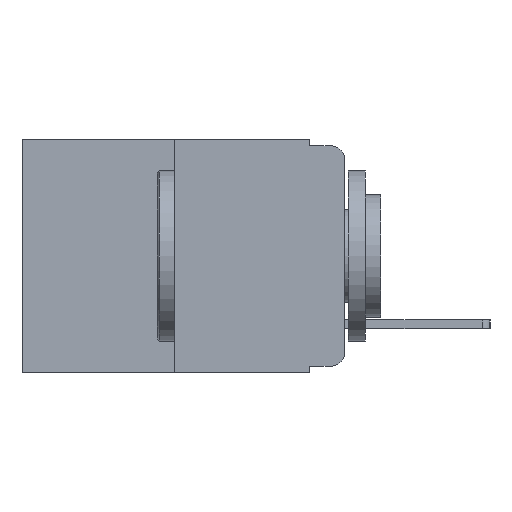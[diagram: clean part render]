
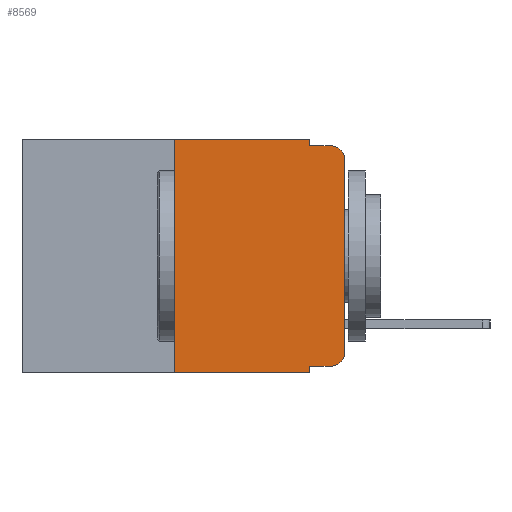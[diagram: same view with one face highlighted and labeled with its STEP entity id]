
A CAD part, left-side view. The second image highlights one B-rep face of the part: STEP entity #8569.
In plain terms, the highlighted planar face has unit normal (-1, 0, 0).
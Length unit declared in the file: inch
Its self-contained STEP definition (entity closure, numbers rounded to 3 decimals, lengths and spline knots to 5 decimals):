
#111 = EDGE_CURVE ( 'NONE', #16404, #5428, #5540, .T. ) ;
#119 = CARTESIAN_POINT ( 'NONE',  ( 0., 0.051, -0.333 ) ) ;
#226 = LINE ( 'NONE', #15794, #16495 ) ;
#444 = LINE ( 'NONE', #6580, #6577 ) ;
#899 = EDGE_CURVE ( 'NONE', #8995, #14313, #8772, .T. ) ;
#959 = DIRECTION ( 'NONE',  ( -1., 0., 0. ) ) ;
#1098 = DIRECTION ( 'NONE',  ( 0., 0., -1. ) ) ;
#1105 = CARTESIAN_POINT ( 'NONE',  ( 0., 0.051, 0. ) ) ;
#1124 = EDGE_CURVE ( 'NONE', #15395, #16404, #5503, .T. ) ;
#1820 = VECTOR ( 'NONE', #13455, 39.37008 ) ;
#2125 = EDGE_CURVE ( 'NONE', #15395, #8322, #14852, .T. ) ;
#2201 = CARTESIAN_POINT ( 'NONE',  ( 0., 0.051, -0.343 ) ) ;
#2273 = AXIS2_PLACEMENT_3D ( 'NONE', #8150, #10680, #2816 ) ;
#2779 = ORIENTED_EDGE ( 'NONE', *, *, #4009, .F. ) ;
#2816 = DIRECTION ( 'NONE',  ( 0., 0., -1. ) ) ;
#3598 = VERTEX_POINT ( 'NONE', #16597 ) ;
#3656 = CARTESIAN_POINT ( 'NONE',  ( 0., 0.25, 0. ) ) ;
#3659 = ORIENTED_EDGE ( 'NONE', *, *, #111, .T. ) ;
#3664 = LINE ( 'NONE', #4885, #10197 ) ;
#3702 = VECTOR ( 'NONE', #17076, 39.37008 ) ;
#4009 = EDGE_CURVE ( 'NONE', #16822, #8995, #16944, .T. ) ;
#4052 = VERTEX_POINT ( 'NONE', #5138 ) ;
#4885 = CARTESIAN_POINT ( 'NONE',  ( 0., 0.051, -0.01 ) ) ;
#4897 = EDGE_CURVE ( 'NONE', #14313, #3598, #11023, .T. ) ;
#5019 = CARTESIAN_POINT ( 'NONE',  ( 0., 0.25, 0. ) ) ;
#5129 = DIRECTION ( 'NONE',  ( 0., -1., 0. ) ) ;
#5138 = CARTESIAN_POINT ( 'NONE',  ( 0., 0., -0.03 ) ) ;
#5311 = VECTOR ( 'NONE', #5129, 39.37008 ) ;
#5428 = VERTEX_POINT ( 'NONE', #6795 ) ;
#5483 = AXIS2_PLACEMENT_3D ( 'NONE', #9072, #959, #10342 ) ;
#5503 = LINE ( 'NONE', #7982, #1820 ) ;
#5540 = CIRCLE ( 'NONE', #11808, 0.02 ) ;
#5636 = CARTESIAN_POINT ( 'NONE',  ( 0., 0.051, 0. ) ) ;
#5819 = EDGE_CURVE ( 'NONE', #3598, #8968, #3664, .T. ) ;
#6263 = DIRECTION ( 'NONE',  ( 0., -1., 0. ) ) ;
#6577 = VECTOR ( 'NONE', #7880, 39.37008 ) ;
#6580 = CARTESIAN_POINT ( 'NONE',  ( 0., 0., 0. ) ) ;
#6795 = CARTESIAN_POINT ( 'NONE',  ( 0., 0., -0.313 ) ) ;
#7580 = EDGE_CURVE ( 'NONE', #4052, #8968, #9988, .T. ) ;
#7582 = FACE_OUTER_BOUND ( 'NONE', #12649, .T. ) ;
#7806 = EDGE_CURVE ( 'NONE', #16822, #8322, #226, .T. ) ;
#7880 = DIRECTION ( 'NONE',  ( 0., 0., 1. ) ) ;
#7950 = CARTESIAN_POINT ( 'NONE',  ( 0., 0.051, 0. ) ) ;
#7982 = CARTESIAN_POINT ( 'NONE',  ( 0., 0.051, -0.333 ) ) ;
#8150 = CARTESIAN_POINT ( 'NONE',  ( 0., 0.473, 0. ) ) ;
#8322 = VERTEX_POINT ( 'NONE', #2201 ) ;
#8329 = CARTESIAN_POINT ( 'NONE',  ( 0., 0.02, -0.333 ) ) ;
#8418 = EDGE_CURVE ( 'NONE', #5428, #4052, #444, .T. ) ;
#8569 = ADVANCED_FACE ( 'NONE', ( #7582 ), #14443, .F. ) ;
#8612 = ORIENTED_EDGE ( 'NONE', *, *, #8418, .T. ) ;
#8772 = LINE ( 'NONE', #9154, #5311 ) ;
#8814 = CARTESIAN_POINT ( 'NONE',  ( 0., 0.02, -0.313 ) ) ;
#8968 = VERTEX_POINT ( 'NONE', #10167 ) ;
#8995 = VERTEX_POINT ( 'NONE', #5019 ) ;
#9072 = CARTESIAN_POINT ( 'NONE',  ( 0., 0.02, -0.03 ) ) ;
#9154 = CARTESIAN_POINT ( 'NONE',  ( 0., 0.473, 0. ) ) ;
#9988 = CIRCLE ( 'NONE', #5483, 0.02 ) ;
#10167 = CARTESIAN_POINT ( 'NONE',  ( 0., 0.02, -0.01 ) ) ;
#10197 = VECTOR ( 'NONE', #6263, 39.37008 ) ;
#10342 = DIRECTION ( 'NONE',  ( 0., 0., -1. ) ) ;
#10680 = DIRECTION ( 'NONE',  ( 1., 0., 0. ) ) ;
#10725 = DIRECTION ( 'NONE',  ( 0., -1., 0. ) ) ;
#11023 = LINE ( 'NONE', #5636, #3702 ) ;
#11109 = VECTOR ( 'NONE', #14367, 39.37008 ) ;
#11732 = CARTESIAN_POINT ( 'NONE',  ( 0., 0.25, -0.343 ) ) ;
#11808 = AXIS2_PLACEMENT_3D ( 'NONE', #8814, #15316, #1098 ) ;
#12379 = ORIENTED_EDGE ( 'NONE', *, *, #7580, .T. ) ;
#12649 = EDGE_LOOP ( 'NONE', ( #8612, #12379, #15716, #12781, #16115, #2779, #13177, #16510, #13581, #3659 ) ) ;
#12781 = ORIENTED_EDGE ( 'NONE', *, *, #4897, .F. ) ;
#13177 = ORIENTED_EDGE ( 'NONE', *, *, #7806, .T. ) ;
#13455 = DIRECTION ( 'NONE',  ( 0., -1., 0. ) ) ;
#13581 = ORIENTED_EDGE ( 'NONE', *, *, #1124, .T. ) ;
#14313 = VERTEX_POINT ( 'NONE', #1105 ) ;
#14367 = DIRECTION ( 'NONE',  ( 0., 0., -1. ) ) ;
#14443 = PLANE ( 'NONE',  #2273 ) ;
#14852 = LINE ( 'NONE', #7950, #11109 ) ;
#15245 = DIRECTION ( 'NONE',  ( 0., 0., 1. ) ) ;
#15316 = DIRECTION ( 'NONE',  ( -1., 0., 0. ) ) ;
#15395 = VERTEX_POINT ( 'NONE', #119 ) ;
#15716 = ORIENTED_EDGE ( 'NONE', *, *, #5819, .F. ) ;
#15794 = CARTESIAN_POINT ( 'NONE',  ( 0., 0.473, -0.343 ) ) ;
#16115 = ORIENTED_EDGE ( 'NONE', *, *, #899, .F. ) ;
#16404 = VERTEX_POINT ( 'NONE', #8329 ) ;
#16495 = VECTOR ( 'NONE', #10725, 39.37008 ) ;
#16510 = ORIENTED_EDGE ( 'NONE', *, *, #2125, .F. ) ;
#16557 = VECTOR ( 'NONE', #15245, 39.37008 ) ;
#16597 = CARTESIAN_POINT ( 'NONE',  ( 0., 0.051, -0.01 ) ) ;
#16822 = VERTEX_POINT ( 'NONE', #11732 ) ;
#16944 = LINE ( 'NONE', #3656, #16557 ) ;
#17076 = DIRECTION ( 'NONE',  ( 0., 0., -1. ) ) ;
